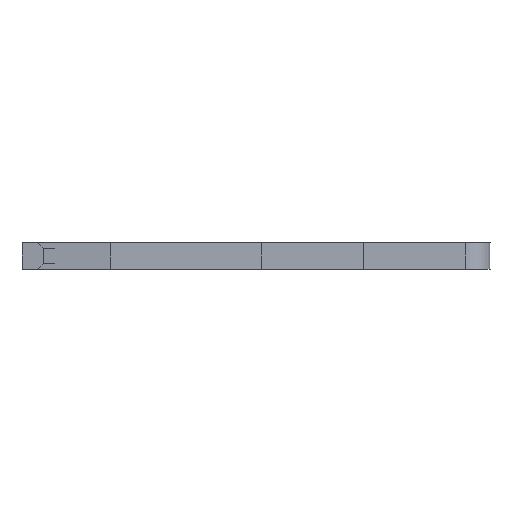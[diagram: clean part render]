
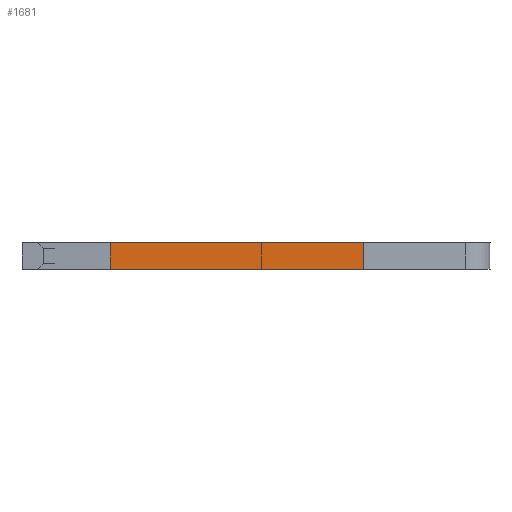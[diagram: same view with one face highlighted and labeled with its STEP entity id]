
A CAD part, left-side view. The second image highlights one B-rep face of the part: STEP entity #1681.
In plain terms, the highlighted face is planar.
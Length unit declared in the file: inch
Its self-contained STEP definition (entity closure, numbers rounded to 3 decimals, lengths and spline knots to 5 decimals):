
#34 = CARTESIAN_POINT ( 'NONE',  ( -0.013, 0.146, -0.0575 ) ) ;
#48 = DIRECTION ( 'NONE',  ( 0., 1., 0. ) ) ;
#183 = AXIS2_PLACEMENT_3D ( 'NONE', #343, #2287, #1003 ) ;
#269 = LINE ( 'NONE', #1773, #1824 ) ;
#271 = LINE ( 'NONE', #1360, #644 ) ;
#301 = EDGE_CURVE ( 'NONE', #891, #2560, #606, .T. ) ;
#305 = ORIENTED_EDGE ( 'NONE', *, *, #301, .F. ) ;
#343 = CARTESIAN_POINT ( 'NONE',  ( 0.013, 0.146, -0.0575 ) ) ;
#378 = VERTEX_POINT ( 'NONE', #874 ) ;
#436 = DIRECTION ( 'NONE',  ( 0., 1., 0. ) ) ;
#528 = EDGE_CURVE ( 'NONE', #891, #378, #271, .T. ) ;
#606 = LINE ( 'NONE', #1086, #1527 ) ;
#644 = VECTOR ( 'NONE', #2612, 39.37008 ) ;
#649 = EDGE_CURVE ( 'NONE', #378, #2526, #1354, .T. ) ;
#741 = EDGE_CURVE ( 'NONE', #2560, #2526, #269, .T. ) ;
#749 = ORIENTED_EDGE ( 'NONE', *, *, #528, .T. ) ;
#874 = CARTESIAN_POINT ( 'NONE',  ( -0.013, -0.099, -0.0575 ) ) ;
#891 = VERTEX_POINT ( 'NONE', #2622 ) ;
#907 = DIRECTION ( 'NONE',  ( -1., 0., 0. ) ) ;
#934 = CARTESIAN_POINT ( 'NONE',  ( -0.013, 0.146, -0.0575 ) ) ;
#1003 = DIRECTION ( 'NONE',  ( 1., 0., 0. ) ) ;
#1086 = CARTESIAN_POINT ( 'NONE',  ( 0.013, 0.146, -0.0575 ) ) ;
#1116 = CARTESIAN_POINT ( 'NONE',  ( 0.013, 0.146, -0.0575 ) ) ;
#1228 = ORIENTED_EDGE ( 'NONE', *, *, #649, .T. ) ;
#1354 = LINE ( 'NONE', #934, #1853 ) ;
#1360 = CARTESIAN_POINT ( 'NONE',  ( 0.013, -0.099, -0.0575 ) ) ;
#1527 = VECTOR ( 'NONE', #436, 39.37008 ) ;
#1681 = ADVANCED_FACE ( 'NONE', ( #2076 ), #2670, .F. ) ;
#1725 = ORIENTED_EDGE ( 'NONE', *, *, #741, .F. ) ;
#1773 = CARTESIAN_POINT ( 'NONE',  ( 0.013, 0.146, -0.0575 ) ) ;
#1824 = VECTOR ( 'NONE', #907, 39.37008 ) ;
#1853 = VECTOR ( 'NONE', #48, 39.37008 ) ;
#2076 = FACE_OUTER_BOUND ( 'NONE', #2589, .T. ) ;
#2287 = DIRECTION ( 'NONE',  ( 0., 0., 1. ) ) ;
#2526 = VERTEX_POINT ( 'NONE', #34 ) ;
#2560 = VERTEX_POINT ( 'NONE', #1116 ) ;
#2589 = EDGE_LOOP ( 'NONE', ( #1228, #1725, #305, #749 ) ) ;
#2612 = DIRECTION ( 'NONE',  ( -1., 0., 0. ) ) ;
#2622 = CARTESIAN_POINT ( 'NONE',  ( 0.013, -0.099, -0.0575 ) ) ;
#2670 = PLANE ( 'NONE',  #183 ) ;
